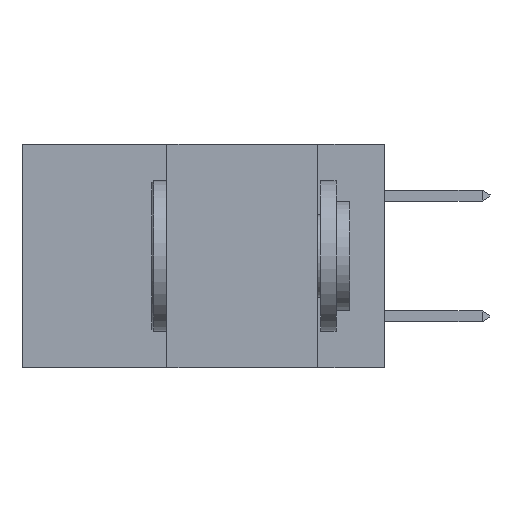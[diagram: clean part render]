
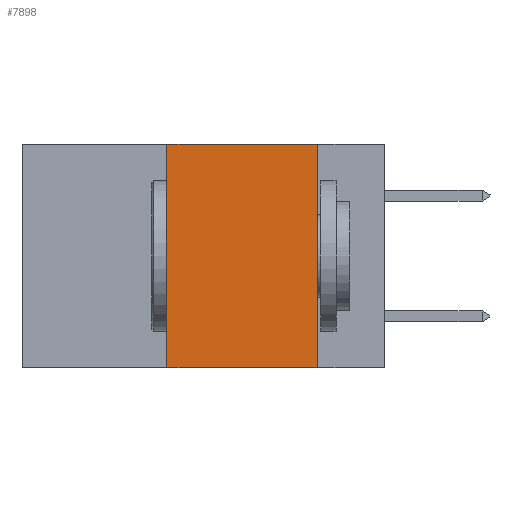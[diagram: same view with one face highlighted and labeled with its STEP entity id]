
A CAD part, left-side view. The second image highlights one B-rep face of the part: STEP entity #7898.
In plain terms, the highlighted planar face has unit normal (-1, 0, 0).
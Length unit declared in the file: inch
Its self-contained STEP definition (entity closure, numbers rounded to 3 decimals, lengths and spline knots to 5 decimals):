
#1276 = EDGE_CURVE ( 'NONE', #26531, #11114, #3394, .T. ) ;
#1402 = CARTESIAN_POINT ( 'NONE',  ( 0., 0.6, 0. ) ) ;
#1719 = VECTOR ( 'NONE', #22727, 39.37008 ) ;
#2130 = VERTEX_POINT ( 'NONE', #27644 ) ;
#3394 = LINE ( 'NONE', #1402, #1719 ) ;
#3919 = VECTOR ( 'NONE', #29897, 39.37008 ) ;
#4148 = EDGE_CURVE ( 'NONE', #11114, #2130, #24777, .T. ) ;
#4622 = CARTESIAN_POINT ( 'NONE',  ( 0., 0.36, 0. ) ) ;
#4858 = DIRECTION ( 'NONE',  ( 0., 0., 1. ) ) ;
#5184 = EDGE_LOOP ( 'NONE', ( #26425, #5852, #27373, #33725 ) ) ;
#5852 = ORIENTED_EDGE ( 'NONE', *, *, #1276, .F. ) ;
#6507 = VERTEX_POINT ( 'NONE', #13593 ) ;
#7590 = CARTESIAN_POINT ( 'NONE',  ( 0., 0.36, 0. ) ) ;
#7898 = ADVANCED_FACE ( 'NONE', ( #13665 ), #13798, .F. ) ;
#7901 = CARTESIAN_POINT ( 'NONE',  ( 0., 0.11, 0. ) ) ;
#10320 = LINE ( 'NONE', #4622, #16163 ) ;
#10930 = DIRECTION ( 'NONE',  ( 0., 0., -1. ) ) ;
#11114 = VERTEX_POINT ( 'NONE', #25198 ) ;
#12288 = EDGE_CURVE ( 'NONE', #6507, #2130, #29756, .T. ) ;
#13593 = CARTESIAN_POINT ( 'NONE',  ( 0., 0.36, -0.37 ) ) ;
#13665 = FACE_OUTER_BOUND ( 'NONE', #5184, .T. ) ;
#13798 = PLANE ( 'NONE',  #29150 ) ;
#16163 = VECTOR ( 'NONE', #4858, 39.37008 ) ;
#18590 = EDGE_CURVE ( 'NONE', #6507, #26531, #10320, .T. ) ;
#18930 = DIRECTION ( 'NONE',  ( 0., 0., -1. ) ) ;
#22692 = VECTOR ( 'NONE', #10930, 39.37008 ) ;
#22727 = DIRECTION ( 'NONE',  ( 0., -1., 0. ) ) ;
#24660 = DIRECTION ( 'NONE',  ( 1., 0., 0. ) ) ;
#24777 = LINE ( 'NONE', #7901, #22692 ) ;
#25198 = CARTESIAN_POINT ( 'NONE',  ( 0., 0.11, 0. ) ) ;
#26425 = ORIENTED_EDGE ( 'NONE', *, *, #4148, .F. ) ;
#26531 = VERTEX_POINT ( 'NONE', #7590 ) ;
#27227 = CARTESIAN_POINT ( 'NONE',  ( 0., 0.6, -0.37 ) ) ;
#27373 = ORIENTED_EDGE ( 'NONE', *, *, #18590, .F. ) ;
#27644 = CARTESIAN_POINT ( 'NONE',  ( 0., 0.11, -0.37 ) ) ;
#29150 = AXIS2_PLACEMENT_3D ( 'NONE', #32728, #24660, #18930 ) ;
#29756 = LINE ( 'NONE', #27227, #3919 ) ;
#29897 = DIRECTION ( 'NONE',  ( 0., -1., 0. ) ) ;
#32728 = CARTESIAN_POINT ( 'NONE',  ( 0., 0.6, 0. ) ) ;
#33725 = ORIENTED_EDGE ( 'NONE', *, *, #12288, .T. ) ;
